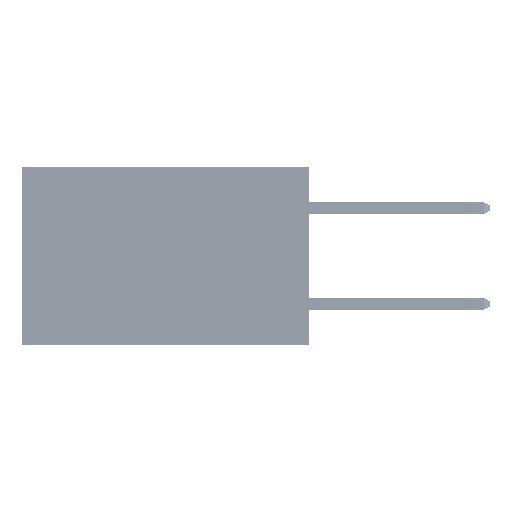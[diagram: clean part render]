
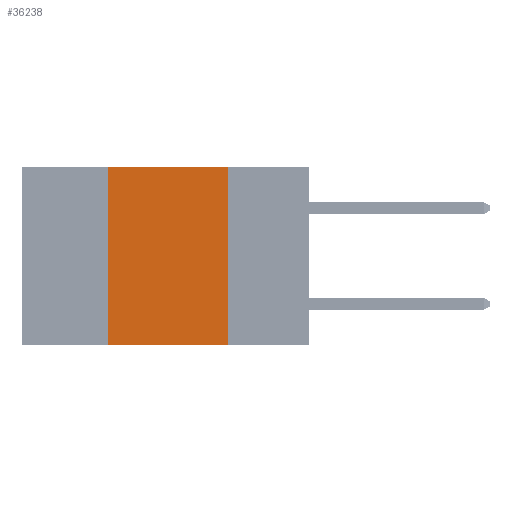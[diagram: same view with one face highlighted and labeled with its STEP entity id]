
A CAD part, left-side view. The second image highlights one B-rep face of the part: STEP entity #36238.
In plain terms, the highlighted planar face has unit normal (-1, 0, 0).
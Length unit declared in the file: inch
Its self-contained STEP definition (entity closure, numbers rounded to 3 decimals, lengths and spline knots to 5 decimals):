
#577 = CARTESIAN_POINT ( 'NONE',  ( 0., 0.17, -0.37 ) ) ;
#923 = CARTESIAN_POINT ( 'NONE',  ( 0., 0.42, 0. ) ) ;
#1239 = EDGE_CURVE ( 'NONE', #39885, #21106, #42956, .T. ) ;
#2111 = ORIENTED_EDGE ( 'NONE', *, *, #11987, .F. ) ;
#4421 = EDGE_CURVE ( 'NONE', #7486, #28113, #21626, .T. ) ;
#7486 = VERTEX_POINT ( 'NONE', #923 ) ;
#10722 = EDGE_LOOP ( 'NONE', ( #33987, #48059, #2111, #41747 ) ) ;
#11130 = LINE ( 'NONE', #44737, #42837 ) ;
#11686 = CARTESIAN_POINT ( 'NONE',  ( 0., 0.6, -0.37 ) ) ;
#11987 = EDGE_CURVE ( 'NONE', #39885, #7486, #11130, .T. ) ;
#12637 = DIRECTION ( 'NONE',  ( 1., 0., 0. ) ) ;
#13725 = CARTESIAN_POINT ( 'NONE',  ( 0., 0.17, 0. ) ) ;
#14637 = FACE_OUTER_BOUND ( 'NONE', #10722, .T. ) ;
#15568 = EDGE_CURVE ( 'NONE', #28113, #21106, #50506, .T. ) ;
#16790 = AXIS2_PLACEMENT_3D ( 'NONE', #32568, #12637, #20915 ) ;
#17270 = VECTOR ( 'NONE', #41185, 39.37008 ) ;
#17536 = DIRECTION ( 'NONE',  ( 0., 0., -1. ) ) ;
#19954 = VECTOR ( 'NONE', #42464, 39.37008 ) ;
#20915 = DIRECTION ( 'NONE',  ( 0., 0., -1. ) ) ;
#21106 = VERTEX_POINT ( 'NONE', #577 ) ;
#21626 = LINE ( 'NONE', #44941, #17270 ) ;
#21956 = DIRECTION ( 'NONE',  ( 0., 0., 1. ) ) ;
#22103 = CARTESIAN_POINT ( 'NONE',  ( 0., 0.42, -0.37 ) ) ;
#28113 = VERTEX_POINT ( 'NONE', #38350 ) ;
#29095 = PLANE ( 'NONE',  #16790 ) ;
#32568 = CARTESIAN_POINT ( 'NONE',  ( 0., 0.6, 0. ) ) ;
#33987 = ORIENTED_EDGE ( 'NONE', *, *, #15568, .F. ) ;
#36238 = ADVANCED_FACE ( 'NONE', ( #14637 ), #29095, .F. ) ;
#38350 = CARTESIAN_POINT ( 'NONE',  ( 0., 0.17, 0. ) ) ;
#39885 = VERTEX_POINT ( 'NONE', #22103 ) ;
#40004 = VECTOR ( 'NONE', #17536, 39.37008 ) ;
#41185 = DIRECTION ( 'NONE',  ( 0., -1., 0. ) ) ;
#41747 = ORIENTED_EDGE ( 'NONE', *, *, #1239, .T. ) ;
#42464 = DIRECTION ( 'NONE',  ( 0., -1., 0. ) ) ;
#42837 = VECTOR ( 'NONE', #21956, 39.37008 ) ;
#42956 = LINE ( 'NONE', #11686, #19954 ) ;
#44737 = CARTESIAN_POINT ( 'NONE',  ( 0., 0.42, 0. ) ) ;
#44941 = CARTESIAN_POINT ( 'NONE',  ( 0., 0.6, 0. ) ) ;
#48059 = ORIENTED_EDGE ( 'NONE', *, *, #4421, .F. ) ;
#50506 = LINE ( 'NONE', #13725, #40004 ) ;
